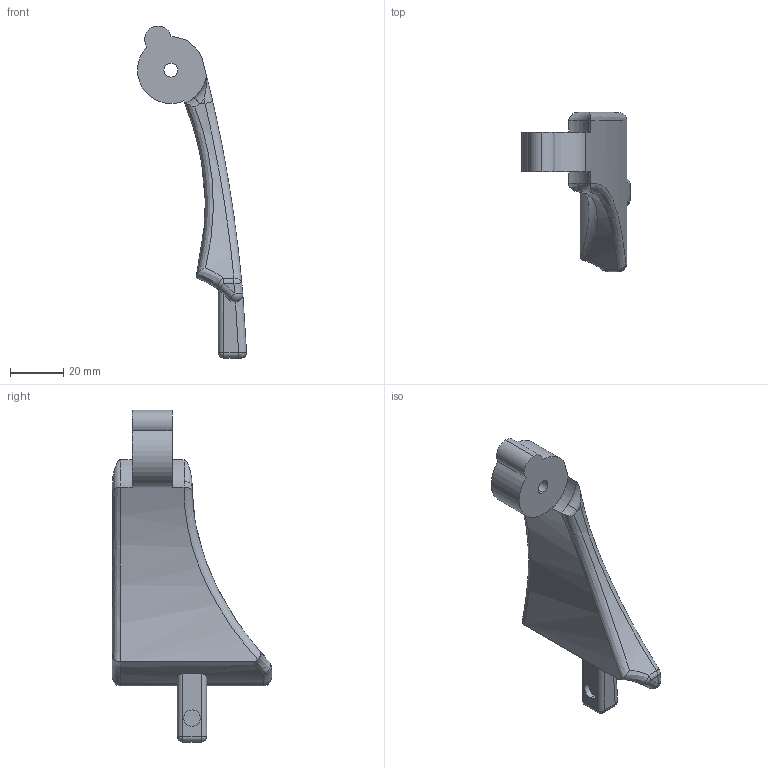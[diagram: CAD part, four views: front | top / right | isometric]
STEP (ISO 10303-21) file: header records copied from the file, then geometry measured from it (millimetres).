
FILE_DESCRIPTION (( 'STEP AP203' ), '1' );
FILE_NAME ('ArmR.STEP', '2020-10-24T03:17:06', ( '' ), ( '' ), 'SwSTEP 2.0', 'SolidWorks 2019', '' );
FILE_SCHEMA (( 'CONFIG_CONTROL_DESIGN' ));
Length unit declared in the file: millimetre
Products named in the file (1): ArmR
Bounding box: 41.08 x 60 x 125.12 mm (x, y, z)
Volume: 45526 mm3; surface area: 12104.1 mm2
Topology: 1 solids, 1 shells, 59 faces, 148 edges, 86 vertices
Faces by surface type: cylinder 24, bspline 15, plane 10, sphere 6, torus 4
Entity records: 2561 total; most frequent: CARTESIAN_POINT 1214, ORIENTED_EDGE 284, DIRECTION 242, EDGE_CURVE 142, AXIS2_PLACEMENT_3D 102, VERTEX_POINT 86, EDGE_LOOP 62, FACE_OUTER_BOUND 59
